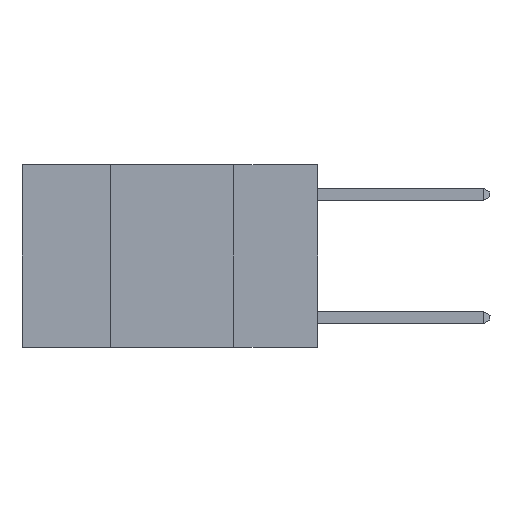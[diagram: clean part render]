
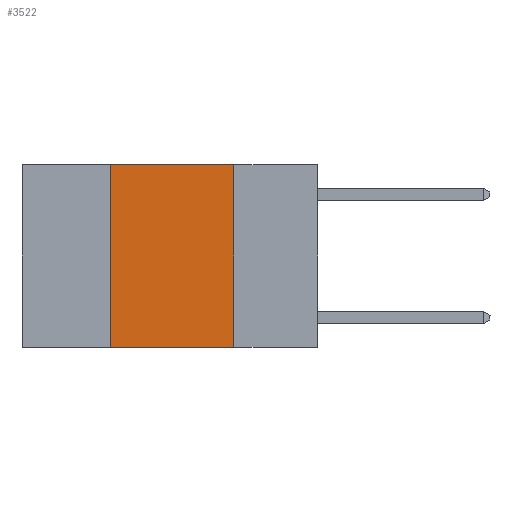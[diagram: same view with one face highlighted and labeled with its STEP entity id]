
A CAD part, left-side view. The second image highlights one B-rep face of the part: STEP entity #3522.
In plain terms, the highlighted planar face has unit normal (-1, 0, 0).
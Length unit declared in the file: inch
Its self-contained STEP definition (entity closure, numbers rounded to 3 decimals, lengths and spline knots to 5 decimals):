
#852 = VECTOR ( 'NONE', #9505, 39.37008 ) ;
#1108 = EDGE_CURVE ( 'NONE', #9890, #4411, #7419, .T. ) ;
#1954 = EDGE_CURVE ( 'NONE', #5496, #9890, #4235, .T. ) ;
#2121 = DIRECTION ( 'NONE',  ( 0., 0., -1. ) ) ;
#2181 = CARTESIAN_POINT ( 'NONE',  ( 0., 0.17, 0. ) ) ;
#2190 = ORIENTED_EDGE ( 'NONE', *, *, #3340, .F. ) ;
#2239 = CARTESIAN_POINT ( 'NONE',  ( 0., 0.42, -0.37 ) ) ;
#2477 = EDGE_CURVE ( 'NONE', #5496, #2801, #5212, .T. ) ;
#2534 = VECTOR ( 'NONE', #2121, 39.37008 ) ;
#2705 = DIRECTION ( 'NONE',  ( 0., -1., 0. ) ) ;
#2801 = VERTEX_POINT ( 'NONE', #8003 ) ;
#2832 = CARTESIAN_POINT ( 'NONE',  ( 0., 0.6, -0.37 ) ) ;
#3340 = EDGE_CURVE ( 'NONE', #4411, #2801, #8819, .T. ) ;
#3522 = ADVANCED_FACE ( 'NONE', ( #7802 ), #9283, .F. ) ;
#3562 = CARTESIAN_POINT ( 'NONE',  ( 0., 0.17, 0. ) ) ;
#3847 = EDGE_LOOP ( 'NONE', ( #2190, #5504, #4633, #4807 ) ) ;
#4235 = LINE ( 'NONE', #7045, #9564 ) ;
#4411 = VERTEX_POINT ( 'NONE', #3562 ) ;
#4633 = ORIENTED_EDGE ( 'NONE', *, *, #1954, .F. ) ;
#4807 = ORIENTED_EDGE ( 'NONE', *, *, #2477, .T. ) ;
#5212 = LINE ( 'NONE', #2832, #6951 ) ;
#5496 = VERTEX_POINT ( 'NONE', #2239 ) ;
#5504 = ORIENTED_EDGE ( 'NONE', *, *, #1108, .F. ) ;
#5922 = CARTESIAN_POINT ( 'NONE',  ( 0., 0.6, 0. ) ) ;
#6951 = VECTOR ( 'NONE', #2705, 39.37008 ) ;
#7010 = CARTESIAN_POINT ( 'NONE',  ( 0., 0.42, 0. ) ) ;
#7045 = CARTESIAN_POINT ( 'NONE',  ( 0., 0.42, 0. ) ) ;
#7419 = LINE ( 'NONE', #5922, #852 ) ;
#7652 = AXIS2_PLACEMENT_3D ( 'NONE', #9332, #9269, #9261 ) ;
#7802 = FACE_OUTER_BOUND ( 'NONE', #3847, .T. ) ;
#8003 = CARTESIAN_POINT ( 'NONE',  ( 0., 0.17, -0.37 ) ) ;
#8819 = LINE ( 'NONE', #2181, #2534 ) ;
#9261 = DIRECTION ( 'NONE',  ( 0., 0., -1. ) ) ;
#9269 = DIRECTION ( 'NONE',  ( 1., 0., 0. ) ) ;
#9283 = PLANE ( 'NONE',  #7652 ) ;
#9332 = CARTESIAN_POINT ( 'NONE',  ( 0., 0.6, 0. ) ) ;
#9505 = DIRECTION ( 'NONE',  ( 0., -1., 0. ) ) ;
#9564 = VECTOR ( 'NONE', #9616, 39.37008 ) ;
#9616 = DIRECTION ( 'NONE',  ( 0., 0., 1. ) ) ;
#9890 = VERTEX_POINT ( 'NONE', #7010 ) ;
